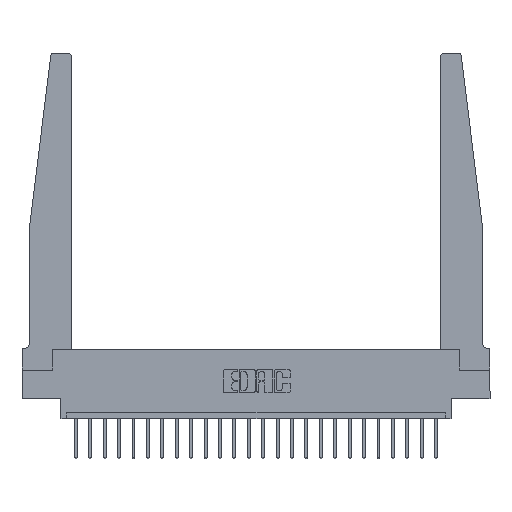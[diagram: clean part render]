
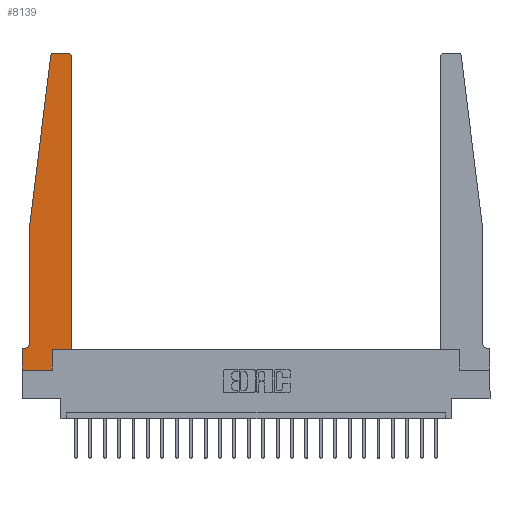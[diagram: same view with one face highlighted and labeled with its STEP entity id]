
A CAD part, top view. The second image highlights one B-rep face of the part: STEP entity #8139.
In plain terms, the highlighted planar face has unit normal (0, 0, 1).
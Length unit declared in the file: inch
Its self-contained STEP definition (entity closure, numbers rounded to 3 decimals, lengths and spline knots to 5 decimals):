
#51 = VECTOR ( 'NONE', #17101, 39.37008 ) ;
#482 = VERTEX_POINT ( 'NONE', #4640 ) ;
#627 = VECTOR ( 'NONE', #13908, 39.37008 ) ;
#849 = LINE ( 'NONE', #17544, #14592 ) ;
#856 = ORIENTED_EDGE ( 'NONE', *, *, #22847, .T. ) ;
#858 = VERTEX_POINT ( 'NONE', #1085 ) ;
#1074 = LINE ( 'NONE', #3071, #20979 ) ;
#1085 = CARTESIAN_POINT ( 'NONE',  ( 0.015, 0.1875, 0.37 ) ) ;
#1904 = CARTESIAN_POINT ( 'NONE',  ( 0.015, 0.2375, 0.37 ) ) ;
#1942 = VERTEX_POINT ( 'NONE', #15924 ) ;
#2059 = DIRECTION ( 'NONE',  ( 0., 0., -1. ) ) ;
#2516 = VERTEX_POINT ( 'NONE', #21998 ) ;
#3071 = CARTESIAN_POINT ( 'NONE',  ( 0., 0., 0.37 ) ) ;
#3125 = LINE ( 'NONE', #14970, #8771 ) ;
#3196 = EDGE_CURVE ( 'NONE', #9646, #10990, #14052, .T. ) ;
#3245 = AXIS2_PLACEMENT_3D ( 'NONE', #1904, #2059, #3714 ) ;
#3524 = CARTESIAN_POINT ( 'NONE',  ( 0., 0., 0.37 ) ) ;
#3714 = DIRECTION ( 'NONE',  ( -1., 0., 0. ) ) ;
#3755 = AXIS2_PLACEMENT_3D ( 'NONE', #22560, #11849, #9977 ) ;
#3985 = DIRECTION ( 'NONE',  ( -1., 0., 0. ) ) ;
#4008 = VERTEX_POINT ( 'NONE', #13464 ) ;
#4459 = ORIENTED_EDGE ( 'NONE', *, *, #16805, .T. ) ;
#4640 = CARTESIAN_POINT ( 'NONE',  ( 0.065, 0.2375, 0.37 ) ) ;
#4828 = AXIS2_PLACEMENT_3D ( 'NONE', #7892, #15063, #14989 ) ;
#6013 = PLANE ( 'NONE',  #11880 ) ;
#6048 = VECTOR ( 'NONE', #3985, 39.37008 ) ;
#6162 = EDGE_LOOP ( 'NONE', ( #22968, #21573, #13977, #15920, #856, #6536, #10894, #16169, #17420, #10715, #15359, #4459 ) ) ;
#6536 = ORIENTED_EDGE ( 'NONE', *, *, #14873, .T. ) ;
#7069 = EDGE_CURVE ( 'NONE', #20291, #4008, #10833, .T. ) ;
#7290 = CARTESIAN_POINT ( 'NONE',  ( 0.2605, 0.18, 0.37 ) ) ;
#7836 = CARTESIAN_POINT ( 'NONE',  ( 0., 0.1875, 0.37 ) ) ;
#7892 = CARTESIAN_POINT ( 'NONE',  ( 0.27653, 2.72, 0.37 ) ) ;
#7998 = LINE ( 'NONE', #3524, #16089 ) ;
#8042 = CARTESIAN_POINT ( 'NONE',  ( 0.425, 0.18, 0.37 ) ) ;
#8139 = ADVANCED_FACE ( 'NONE', ( #17225 ), #6013, .T. ) ;
#8566 = CARTESIAN_POINT ( 'NONE',  ( 0.065, 1.25, 0.37 ) ) ;
#8771 = VECTOR ( 'NONE', #15217, 39.37008 ) ;
#8815 = CARTESIAN_POINT ( 'NONE',  ( 0.065, 1.25, 0.37 ) ) ;
#9191 = LINE ( 'NONE', #7290, #18695 ) ;
#9405 = VERTEX_POINT ( 'NONE', #15622 ) ;
#9511 = DIRECTION ( 'NONE',  ( 0., 1., 0. ) ) ;
#9646 = VERTEX_POINT ( 'NONE', #14501 ) ;
#9784 = DIRECTION ( 'NONE',  ( 0., 0., 1. ) ) ;
#9931 = EDGE_CURVE ( 'NONE', #13684, #482, #16298, .T. ) ;
#9977 = DIRECTION ( 'NONE',  ( 1., 0., 0. ) ) ;
#10078 = VECTOR ( 'NONE', #9511, 39.37008 ) ;
#10715 = ORIENTED_EDGE ( 'NONE', *, *, #3196, .T. ) ;
#10833 = CIRCLE ( 'NONE', #4828, 0.03 ) ;
#10894 = ORIENTED_EDGE ( 'NONE', *, *, #12284, .T. ) ;
#10990 = VERTEX_POINT ( 'NONE', #8042 ) ;
#11079 = EDGE_CURVE ( 'NONE', #9405, #20291, #849, .T. ) ;
#11265 = VERTEX_POINT ( 'NONE', #14050 ) ;
#11591 = CIRCLE ( 'NONE', #3245, 0.05 ) ;
#11841 = CIRCLE ( 'NONE', #3755, 0.03 ) ;
#11849 = DIRECTION ( 'NONE',  ( 0., 0., 1. ) ) ;
#11880 = AXIS2_PLACEMENT_3D ( 'NONE', #7836, #9784, #20341 ) ;
#11958 = CARTESIAN_POINT ( 'NONE',  ( 0.27653, 2.75, 0.37 ) ) ;
#12195 = DIRECTION ( 'NONE',  ( -1., 0., 0. ) ) ;
#12284 = EDGE_CURVE ( 'NONE', #1942, #12567, #1074, .T. ) ;
#12567 = VERTEX_POINT ( 'NONE', #15647 ) ;
#12610 = CARTESIAN_POINT ( 'NONE',  ( 0.065, 0.1875, 0.37 ) ) ;
#13464 = CARTESIAN_POINT ( 'NONE',  ( 0.24675, 2.72367, 0.37 ) ) ;
#13592 = LINE ( 'NONE', #12610, #6048 ) ;
#13684 = VERTEX_POINT ( 'NONE', #8815 ) ;
#13908 = DIRECTION ( 'NONE',  ( 0., -1., 0. ) ) ;
#13977 = ORIENTED_EDGE ( 'NONE', *, *, #17176, .T. ) ;
#14050 = CARTESIAN_POINT ( 'NONE',  ( 0.2605, 0., 0.37 ) ) ;
#14052 = LINE ( 'NONE', #19830, #51 ) ;
#14501 = CARTESIAN_POINT ( 'NONE',  ( 0.2605, 0.18, 0.37 ) ) ;
#14592 = VECTOR ( 'NONE', #12195, 39.37008 ) ;
#14594 = DIRECTION ( 'NONE',  ( 0., -1., 0. ) ) ;
#14873 = EDGE_CURVE ( 'NONE', #858, #1942, #13592, .T. ) ;
#14970 = CARTESIAN_POINT ( 'NONE',  ( 0.065, 1.25, 0.37 ) ) ;
#14989 = DIRECTION ( 'NONE',  ( 1., 0., 0. ) ) ;
#15063 = DIRECTION ( 'NONE',  ( 0., 0., 1. ) ) ;
#15217 = DIRECTION ( 'NONE',  ( -0.122, -0.992, 0. ) ) ;
#15359 = ORIENTED_EDGE ( 'NONE', *, *, #18736, .T. ) ;
#15622 = CARTESIAN_POINT ( 'NONE',  ( 0.395, 2.75, 0.37 ) ) ;
#15647 = CARTESIAN_POINT ( 'NONE',  ( 0., 0., 0.37 ) ) ;
#15920 = ORIENTED_EDGE ( 'NONE', *, *, #9931, .T. ) ;
#15924 = CARTESIAN_POINT ( 'NONE',  ( 0., 0.1875, 0.37 ) ) ;
#16043 = EDGE_CURVE ( 'NONE', #12567, #11265, #7998, .T. ) ;
#16089 = VECTOR ( 'NONE', #16090, 39.37008 ) ;
#16090 = DIRECTION ( 'NONE',  ( 1., 0., 0. ) ) ;
#16169 = ORIENTED_EDGE ( 'NONE', *, *, #16043, .T. ) ;
#16212 = DIRECTION ( 'NONE',  ( 0., 1., 0. ) ) ;
#16298 = LINE ( 'NONE', #8566, #627 ) ;
#16805 = EDGE_CURVE ( 'NONE', #2516, #9405, #11841, .T. ) ;
#17101 = DIRECTION ( 'NONE',  ( 1., 0., 0. ) ) ;
#17176 = EDGE_CURVE ( 'NONE', #4008, #13684, #3125, .T. ) ;
#17225 = FACE_OUTER_BOUND ( 'NONE', #6162, .T. ) ;
#17420 = ORIENTED_EDGE ( 'NONE', *, *, #19944, .T. ) ;
#17544 = CARTESIAN_POINT ( 'NONE',  ( 0.25, 2.75, 0.37 ) ) ;
#18695 = VECTOR ( 'NONE', #16212, 39.37008 ) ;
#18736 = EDGE_CURVE ( 'NONE', #10990, #2516, #19038, .T. ) ;
#19038 = LINE ( 'NONE', #20217, #10078 ) ;
#19830 = CARTESIAN_POINT ( 'NONE',  ( 0.425, 0.18, 0.37 ) ) ;
#19944 = EDGE_CURVE ( 'NONE', #11265, #9646, #9191, .T. ) ;
#20217 = CARTESIAN_POINT ( 'NONE',  ( 0.425, 0.18, 0.37 ) ) ;
#20291 = VERTEX_POINT ( 'NONE', #11958 ) ;
#20341 = DIRECTION ( 'NONE',  ( 1., 0., 0. ) ) ;
#20979 = VECTOR ( 'NONE', #14594, 39.37008 ) ;
#21573 = ORIENTED_EDGE ( 'NONE', *, *, #7069, .T. ) ;
#21998 = CARTESIAN_POINT ( 'NONE',  ( 0.425, 2.72, 0.37 ) ) ;
#22560 = CARTESIAN_POINT ( 'NONE',  ( 0.395, 2.72, 0.37 ) ) ;
#22847 = EDGE_CURVE ( 'NONE', #482, #858, #11591, .T. ) ;
#22968 = ORIENTED_EDGE ( 'NONE', *, *, #11079, .T. ) ;
